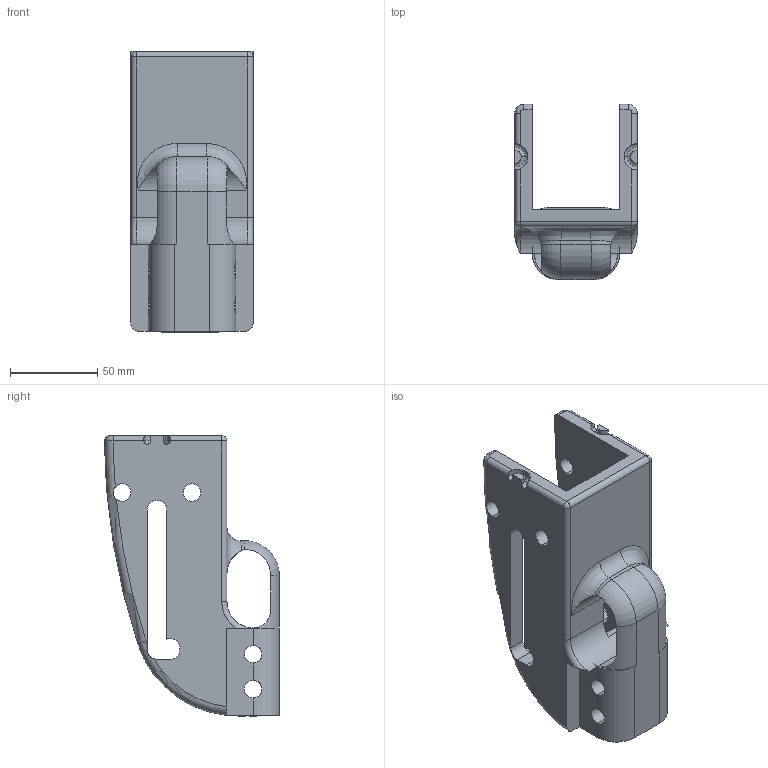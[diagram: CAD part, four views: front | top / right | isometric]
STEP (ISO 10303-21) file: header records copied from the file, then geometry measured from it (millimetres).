
FILE_DESCRIPTION (( 'STEP AP203' ), '1' );
FILE_NAME ('Body.STEP', '2013-08-28T12:52:11', ( '' ), ( '' ), 'SwSTEP 2.0', 'SolidWorks 2013', '' );
FILE_SCHEMA (( 'CONFIG_CONTROL_DESIGN' ));
Length unit declared in the file: millimetre
Products named in the file (1): Body
Bounding box: 70 x 99.99 x 160.5 mm (x, y, z)
Volume: 300957.1 mm3; surface area: 72401 mm2
Topology: 1 solids, 1 shells, 783 faces, 2274 edges, 1498 vertices
Faces by surface type: bspline 592, plane 113, cylinder 61, torus 15, sphere 2
Entity records: 38644 total; most frequent: CARTESIAN_POINT 21960, ORIENTED_EDGE 4544, EDGE_CURVE 2272, DIRECTION 1583, VERTEX_POINT 1498, B_SPLINE_CURVE_WITH_KNOTS 1206, LINE 925, VECTOR 925
